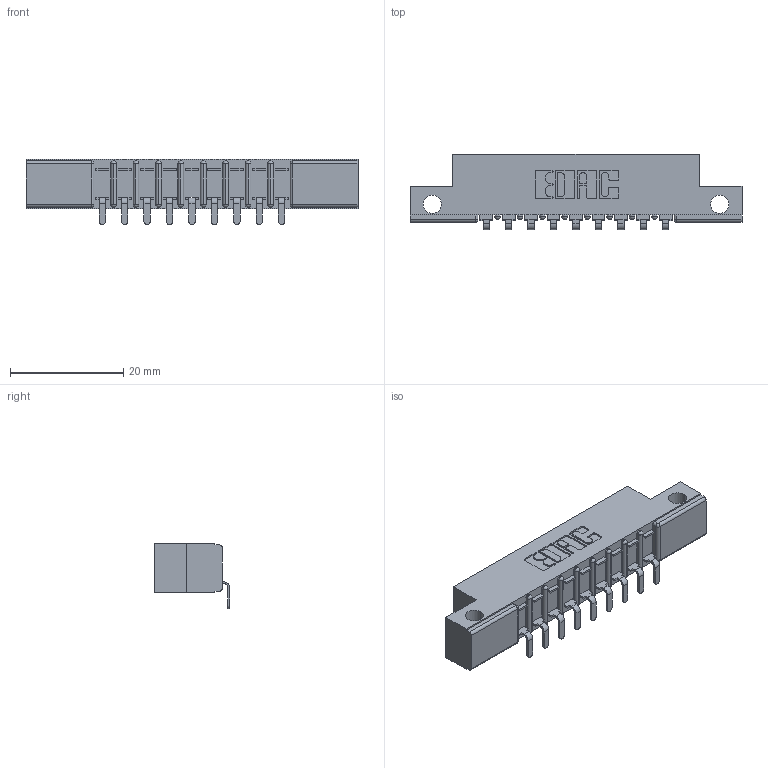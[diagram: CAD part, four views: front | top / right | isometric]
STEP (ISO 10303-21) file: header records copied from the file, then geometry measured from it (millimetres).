
FILE_DESCRIPTION (( 'STEP AP203' ), '1' );
FILE_NAME ('357-009-553-112.STEP', '2018-08-07T02:12:03', ( '' ), ( '' ), 'SwSTEP 2.0', 'SolidWorks 2016', '' );
FILE_SCHEMA (( 'CONFIG_CONTROL_DESIGN' ));
Length unit declared in the file: inch
Products named in the file (3): 307 Part_.128 Dia Side Mounting Holes; 307-290-002_553; 357-009-553-112
Assembly tree (10 placements, depth 2):
  357-009-553-112
    307 Part_.128 Dia Side Mounting Holes
    307-290-002_553  x9
Bounding box: 58.67 x 13.32 x 11.51 mm (x, y, z)
Volume: 3790.8 mm3; surface area: 6037.1 mm2
Topology: 10 solids, 10 shells, 830 faces, 2519 edges, 1650 vertices
Faces by surface type: plane 493, cylinder 317, sphere 20
Entity records: 12640 total; most frequent: CARTESIAN_POINT 2128, ORIENTED_EDGE 2118, DIRECTION 2083, EDGE_CURVE 1059, VECTOR 793, LINE 793, VERTEX_POINT 690, AXIS2_PLACEMENT_3D 645
